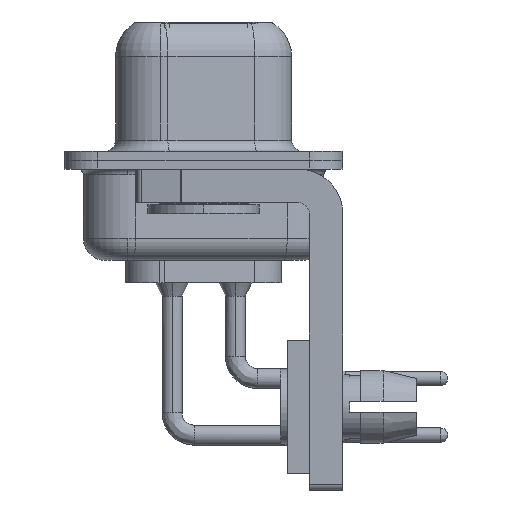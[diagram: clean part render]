
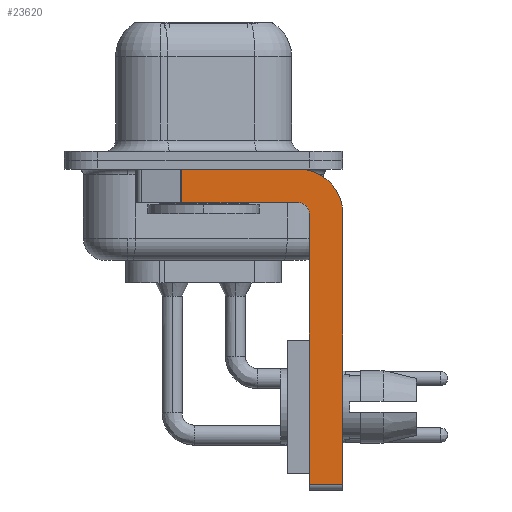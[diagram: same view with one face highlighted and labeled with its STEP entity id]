
A CAD part, left-side view. The second image highlights one B-rep face of the part: STEP entity #23620.
In plain terms, the highlighted planar face has unit normal (-1, 0, 0).
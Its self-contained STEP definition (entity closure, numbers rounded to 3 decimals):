
#119 = VECTOR ( 'NONE', #14703, 1000. ) ;
#154 = VECTOR ( 'NONE', #30494, 1000. ) ;
#699 = VERTEX_POINT ( 'NONE', #13312 ) ;
#895 = LINE ( 'NONE', #22165, #119 ) ;
#1251 = EDGE_CURVE ( 'NONE', #13622, #11215, #7384, .T. ) ;
#1378 = CARTESIAN_POINT ( 'NONE',  ( -2.9, -4.25, -2.4 ) ) ;
#1444 = DIRECTION ( 'NONE',  ( 1., 0., 0. ) ) ;
#1633 = ORIENTED_EDGE ( 'NONE', *, *, #13292, .F. ) ;
#2037 = EDGE_CURVE ( 'NONE', #24589, #27708, #13614, .T. ) ;
#2508 = ORIENTED_EDGE ( 'NONE', *, *, #1251, .T. ) ;
#2751 = FACE_OUTER_BOUND ( 'NONE', #19380, .T. ) ;
#3663 = VECTOR ( 'NONE', #6116, 1000. ) ;
#3901 = DIRECTION ( 'NONE',  ( 0., 0., 1. ) ) ;
#5396 = EDGE_CURVE ( 'NONE', #18381, #27708, #19895, .T. ) ;
#6116 = DIRECTION ( 'NONE',  ( 0., 0., 1. ) ) ;
#7384 = LINE ( 'NONE', #27238, #20572 ) ;
#11215 = VERTEX_POINT ( 'NONE', #27488 ) ;
#11304 = EDGE_CURVE ( 'NONE', #13622, #699, #11958, .T. ) ;
#11405 = EDGE_CURVE ( 'NONE', #699, #18381, #15490, .T. ) ;
#11427 = CARTESIAN_POINT ( 'NONE',  ( -2.9, -4.25, -1.9 ) ) ;
#11452 = ORIENTED_EDGE ( 'NONE', *, *, #5396, .F. ) ;
#11958 = LINE ( 'NONE', #20521, #154 ) ;
#12937 = AXIS2_PLACEMENT_3D ( 'NONE', #13536, #30813, #16046 ) ;
#13205 = CARTESIAN_POINT ( 'NONE',  ( -2.9, -4.75, -14.55 ) ) ;
#13292 = EDGE_CURVE ( 'NONE', #19061, #14610, #22521, .T. ) ;
#13312 = CARTESIAN_POINT ( 'NONE',  ( -2.9, -4.25, -0.4 ) ) ;
#13352 = VECTOR ( 'NONE', #24833, 1000. ) ;
#13536 = CARTESIAN_POINT ( 'NONE',  ( -2.9, -4.25, -2.4 ) ) ;
#13614 = LINE ( 'NONE', #31284, #25833 ) ;
#13622 = VERTEX_POINT ( 'NONE', #22262 ) ;
#14076 = AXIS2_PLACEMENT_3D ( 'NONE', #1378, #18911, #3901 ) ;
#14610 = VERTEX_POINT ( 'NONE', #11427 ) ;
#14703 = DIRECTION ( 'NONE',  ( 0., 1., 0. ) ) ;
#15490 = CIRCLE ( 'NONE', #12937, 2. ) ;
#16046 = DIRECTION ( 'NONE',  ( 0., 0., -1. ) ) ;
#16523 = PLANE ( 'NONE',  #20747 ) ;
#17047 = LINE ( 'NONE', #28321, #3663 ) ;
#17469 = EDGE_CURVE ( 'NONE', #24589, #19061, #17047, .T. ) ;
#18348 = ORIENTED_EDGE ( 'NONE', *, *, #2037, .T. ) ;
#18381 = VERTEX_POINT ( 'NONE', #21563 ) ;
#18911 = DIRECTION ( 'NONE',  ( -1., 0., 0. ) ) ;
#18975 = DIRECTION ( 'NONE',  ( 0., 0., -1. ) ) ;
#19061 = VERTEX_POINT ( 'NONE', #19828 ) ;
#19380 = EDGE_LOOP ( 'NONE', ( #21731, #2508, #24739, #1633, #29547, #18348, #11452, #26094 ) ) ;
#19828 = CARTESIAN_POINT ( 'NONE',  ( -2.9, -4.75, -2.4 ) ) ;
#19844 = DIRECTION ( 'NONE',  ( 0., -1., 0. ) ) ;
#19895 = LINE ( 'NONE', #24940, #13352 ) ;
#20521 = CARTESIAN_POINT ( 'NONE',  ( -2.9, 3., -0.4 ) ) ;
#20572 = VECTOR ( 'NONE', #25164, 1000. ) ;
#20747 = AXIS2_PLACEMENT_3D ( 'NONE', #28755, #1444, #18975 ) ;
#21563 = CARTESIAN_POINT ( 'NONE',  ( -2.9, -6.25, -2.4 ) ) ;
#21731 = ORIENTED_EDGE ( 'NONE', *, *, #11304, .F. ) ;
#22165 = CARTESIAN_POINT ( 'NONE',  ( -2.9, -4.25, -1.9 ) ) ;
#22262 = CARTESIAN_POINT ( 'NONE',  ( -2.9, 0.978, -0.4 ) ) ;
#22521 = CIRCLE ( 'NONE', #14076, 0.5 ) ;
#23620 = ADVANCED_FACE ( 'NONE', ( #2751 ), #16523, .F. ) ;
#24589 = VERTEX_POINT ( 'NONE', #13205 ) ;
#24739 = ORIENTED_EDGE ( 'NONE', *, *, #28804, .F. ) ;
#24833 = DIRECTION ( 'NONE',  ( 0., 0., -1. ) ) ;
#24940 = CARTESIAN_POINT ( 'NONE',  ( -2.9, -6.25, -2.4 ) ) ;
#25164 = DIRECTION ( 'NONE',  ( 0., 0., -1. ) ) ;
#25833 = VECTOR ( 'NONE', #19844, 1000. ) ;
#26094 = ORIENTED_EDGE ( 'NONE', *, *, #11405, .F. ) ;
#27238 = CARTESIAN_POINT ( 'NONE',  ( -2.9, 0.978, -1.9 ) ) ;
#27488 = CARTESIAN_POINT ( 'NONE',  ( -2.9, 0.978, -1.9 ) ) ;
#27708 = VERTEX_POINT ( 'NONE', #30625 ) ;
#28321 = CARTESIAN_POINT ( 'NONE',  ( -2.9, -4.75, -14.8 ) ) ;
#28755 = CARTESIAN_POINT ( 'NONE',  ( -2.9, -4.25, -2.4 ) ) ;
#28804 = EDGE_CURVE ( 'NONE', #14610, #11215, #895, .T. ) ;
#29547 = ORIENTED_EDGE ( 'NONE', *, *, #17469, .F. ) ;
#30494 = DIRECTION ( 'NONE',  ( 0., -1., 0. ) ) ;
#30625 = CARTESIAN_POINT ( 'NONE',  ( -2.9, -6.25, -14.55 ) ) ;
#30813 = DIRECTION ( 'NONE',  ( 1., 0., 0. ) ) ;
#31284 = CARTESIAN_POINT ( 'NONE',  ( -2.9, -4.25, -14.55 ) ) ;
